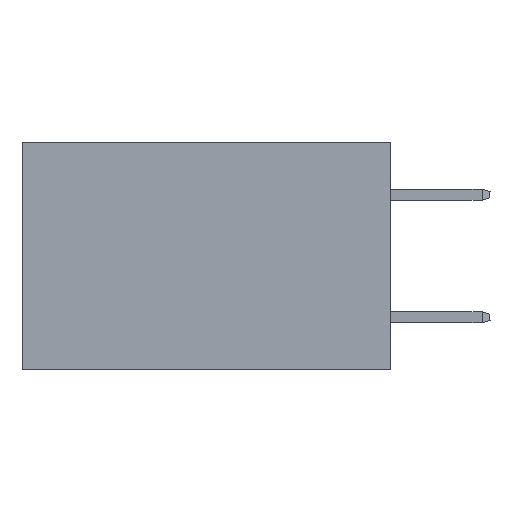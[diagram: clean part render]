
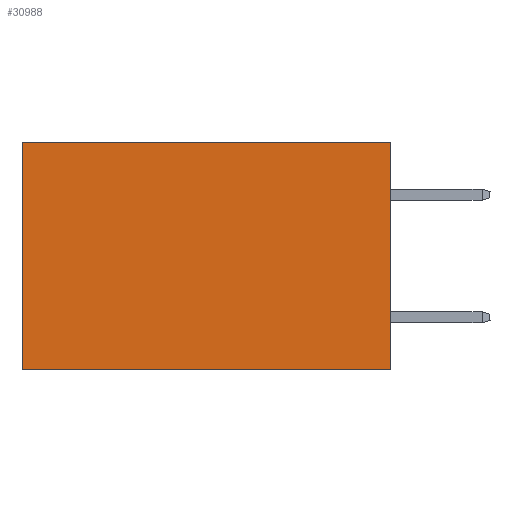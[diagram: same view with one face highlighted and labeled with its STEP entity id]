
A CAD part, left-side view. The second image highlights one B-rep face of the part: STEP entity #30988.
In plain terms, the highlighted planar face has unit normal (-1, 0, 0).
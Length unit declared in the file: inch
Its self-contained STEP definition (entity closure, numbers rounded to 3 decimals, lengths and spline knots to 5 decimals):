
#606 = EDGE_CURVE ( 'NONE', #29002, #29256, #29880, .T. ) ;
#944 = LINE ( 'NONE', #17258, #29397 ) ;
#2400 = ORIENTED_EDGE ( 'NONE', *, *, #8608, .F. ) ;
#2809 = PLANE ( 'NONE',  #4496 ) ;
#4496 = AXIS2_PLACEMENT_3D ( 'NONE', #8439, #28954, #32020 ) ;
#5089 = CARTESIAN_POINT ( 'NONE',  ( 0.2875, 0., 0. ) ) ;
#5484 = VECTOR ( 'NONE', #21878, 39.37008 ) ;
#5803 = VERTEX_POINT ( 'NONE', #20244 ) ;
#8439 = CARTESIAN_POINT ( 'NONE',  ( 0.2875, 0., 0. ) ) ;
#8608 = EDGE_CURVE ( 'NONE', #5803, #29002, #944, .T. ) ;
#10585 = CARTESIAN_POINT ( 'NONE',  ( 0.2875, 0., -0.37 ) ) ;
#10590 = ORIENTED_EDGE ( 'NONE', *, *, #31360, .T. ) ;
#12851 = VECTOR ( 'NONE', #31392, 39.37008 ) ;
#12924 = ORIENTED_EDGE ( 'NONE', *, *, #37280, .T. ) ;
#13138 = ORIENTED_EDGE ( 'NONE', *, *, #606, .F. ) ;
#16568 = FACE_OUTER_BOUND ( 'NONE', #27768, .T. ) ;
#17258 = CARTESIAN_POINT ( 'NONE',  ( 0.2875, 0., 0. ) ) ;
#18809 = CARTESIAN_POINT ( 'NONE',  ( 0.2875, 0., -0.37 ) ) ;
#18863 = LINE ( 'NONE', #33065, #5484 ) ;
#19149 = CARTESIAN_POINT ( 'NONE',  ( 0.2875, 0.6, 0. ) ) ;
#20244 = CARTESIAN_POINT ( 'NONE',  ( 0.2875, 0., 0. ) ) ;
#20664 = LINE ( 'NONE', #5089, #12851 ) ;
#21878 = DIRECTION ( 'NONE',  ( 0., 0., -1. ) ) ;
#22977 = VECTOR ( 'NONE', #34972, 39.37008 ) ;
#24730 = VERTEX_POINT ( 'NONE', #19149 ) ;
#27768 = EDGE_LOOP ( 'NONE', ( #10590, #13138, #2400, #12924 ) ) ;
#28954 = DIRECTION ( 'NONE',  ( 1., 0., 0. ) ) ;
#29002 = VERTEX_POINT ( 'NONE', #18809 ) ;
#29256 = VERTEX_POINT ( 'NONE', #34405 ) ;
#29397 = VECTOR ( 'NONE', #29568, 39.37008 ) ;
#29568 = DIRECTION ( 'NONE',  ( 0., 0., -1. ) ) ;
#29880 = LINE ( 'NONE', #10585, #22977 ) ;
#30988 = ADVANCED_FACE ( 'NONE', ( #16568 ), #2809, .F. ) ;
#31360 = EDGE_CURVE ( 'NONE', #24730, #29256, #18863, .T. ) ;
#31392 = DIRECTION ( 'NONE',  ( 0., 1., 0. ) ) ;
#32020 = DIRECTION ( 'NONE',  ( 0., 0., -1. ) ) ;
#33065 = CARTESIAN_POINT ( 'NONE',  ( 0.2875, 0.6, 0. ) ) ;
#34405 = CARTESIAN_POINT ( 'NONE',  ( 0.2875, 0.6, -0.37 ) ) ;
#34972 = DIRECTION ( 'NONE',  ( 0., 1., 0. ) ) ;
#37280 = EDGE_CURVE ( 'NONE', #5803, #24730, #20664, .T. ) ;
